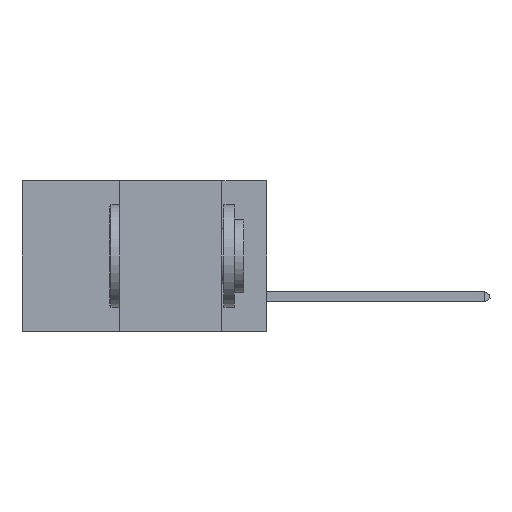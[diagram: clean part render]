
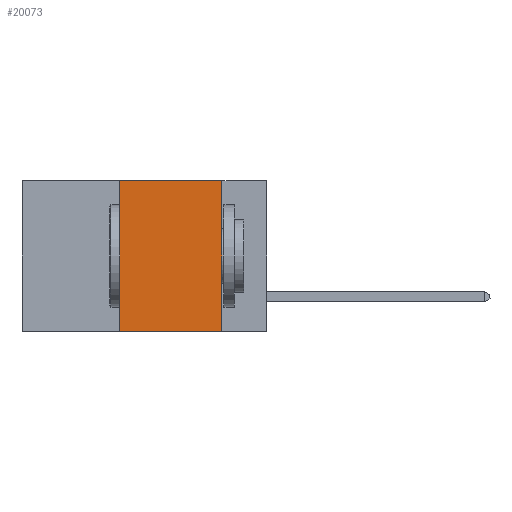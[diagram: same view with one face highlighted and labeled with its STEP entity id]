
A CAD part, left-side view. The second image highlights one B-rep face of the part: STEP entity #20073.
In plain terms, the highlighted planar face has unit normal (-1, 0, 0).
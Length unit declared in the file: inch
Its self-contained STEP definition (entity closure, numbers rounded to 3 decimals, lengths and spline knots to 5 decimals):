
#284 = LINE ( 'NONE', #16106, #8981 ) ;
#1170 = VECTOR ( 'NONE', #14881, 39.37008 ) ;
#1458 = EDGE_CURVE ( 'NONE', #13162, #1570, #284, .T. ) ;
#1488 = EDGE_CURVE ( 'NONE', #12102, #2822, #12928, .T. ) ;
#1570 = VERTEX_POINT ( 'NONE', #14090 ) ;
#1714 = LINE ( 'NONE', #4639, #1170 ) ;
#2415 = CARTESIAN_POINT ( 'NONE',  ( 0., 0.11, -0.37 ) ) ;
#2822 = VERTEX_POINT ( 'NONE', #2415 ) ;
#4313 = CARTESIAN_POINT ( 'NONE',  ( 0., 0.36, -0.37 ) ) ;
#4613 = LINE ( 'NONE', #13680, #8718 ) ;
#4639 = CARTESIAN_POINT ( 'NONE',  ( 0., 0.36, 0. ) ) ;
#5171 = FACE_OUTER_BOUND ( 'NONE', #8700, .T. ) ;
#6311 = AXIS2_PLACEMENT_3D ( 'NONE', #20205, #10237, #21815 ) ;
#8535 = PLANE ( 'NONE',  #6311 ) ;
#8700 = EDGE_LOOP ( 'NONE', ( #17571, #13809, #11354, #12439 ) ) ;
#8718 = VECTOR ( 'NONE', #15362, 39.37008 ) ;
#8981 = VECTOR ( 'NONE', #15945, 39.37008 ) ;
#10237 = DIRECTION ( 'NONE',  ( 1., 0., 0. ) ) ;
#11354 = ORIENTED_EDGE ( 'NONE', *, *, #19243, .F. ) ;
#12102 = VERTEX_POINT ( 'NONE', #4313 ) ;
#12439 = ORIENTED_EDGE ( 'NONE', *, *, #1488, .T. ) ;
#12458 = CARTESIAN_POINT ( 'NONE',  ( 0., 0.36, 0. ) ) ;
#12928 = LINE ( 'NONE', #15642, #13461 ) ;
#13162 = VERTEX_POINT ( 'NONE', #12458 ) ;
#13461 = VECTOR ( 'NONE', #15710, 39.37008 ) ;
#13680 = CARTESIAN_POINT ( 'NONE',  ( 0., 0.11, 0. ) ) ;
#13809 = ORIENTED_EDGE ( 'NONE', *, *, #1458, .F. ) ;
#14090 = CARTESIAN_POINT ( 'NONE',  ( 0., 0.11, 0. ) ) ;
#14881 = DIRECTION ( 'NONE',  ( 0., 0., 1. ) ) ;
#15362 = DIRECTION ( 'NONE',  ( 0., 0., -1. ) ) ;
#15642 = CARTESIAN_POINT ( 'NONE',  ( 0., 0.6, -0.37 ) ) ;
#15710 = DIRECTION ( 'NONE',  ( 0., -1., 0. ) ) ;
#15945 = DIRECTION ( 'NONE',  ( 0., -1., 0. ) ) ;
#16106 = CARTESIAN_POINT ( 'NONE',  ( 0., 0.6, 0. ) ) ;
#17571 = ORIENTED_EDGE ( 'NONE', *, *, #20103, .F. ) ;
#19243 = EDGE_CURVE ( 'NONE', #12102, #13162, #1714, .T. ) ;
#20073 = ADVANCED_FACE ( 'NONE', ( #5171 ), #8535, .F. ) ;
#20103 = EDGE_CURVE ( 'NONE', #1570, #2822, #4613, .T. ) ;
#20205 = CARTESIAN_POINT ( 'NONE',  ( 0., 0.6, 0. ) ) ;
#21815 = DIRECTION ( 'NONE',  ( 0., 0., -1. ) ) ;
